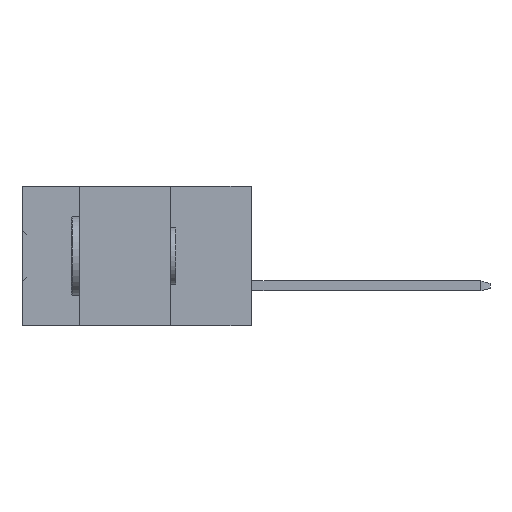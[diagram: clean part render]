
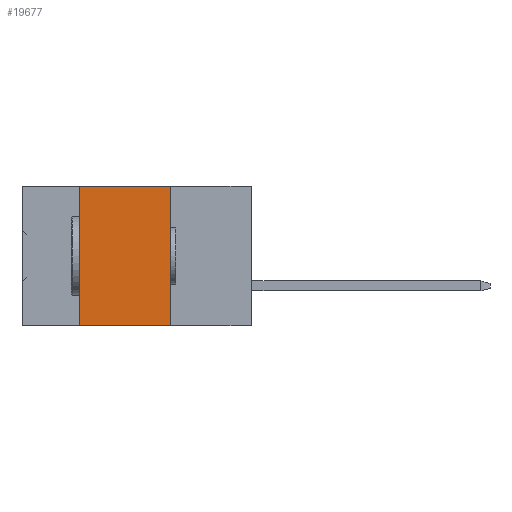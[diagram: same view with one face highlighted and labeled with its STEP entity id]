
A CAD part, left-side view. The second image highlights one B-rep face of the part: STEP entity #19677.
In plain terms, the highlighted planar face has unit normal (-1, 0, 0).
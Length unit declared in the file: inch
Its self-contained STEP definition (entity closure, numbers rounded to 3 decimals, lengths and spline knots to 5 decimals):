
#2339 = CARTESIAN_POINT ( 'NONE',  ( 0., 0.54, 0. ) ) ;
#2583 = AXIS2_PLACEMENT_3D ( 'NONE', #28787, #11927, #6808 ) ;
#3041 = CARTESIAN_POINT ( 'NONE',  ( 0., 0.54, -0.437 ) ) ;
#3697 = DIRECTION ( 'NONE',  ( 0., -1., 0. ) ) ;
#3862 = CARTESIAN_POINT ( 'NONE',  ( 0., 0.72, 0. ) ) ;
#4783 = LINE ( 'NONE', #19678, #19784 ) ;
#5439 = EDGE_CURVE ( 'NONE', #28182, #17520, #30820, .T. ) ;
#6808 = DIRECTION ( 'NONE',  ( 0., 0., -1. ) ) ;
#7467 = VERTEX_POINT ( 'NONE', #27757 ) ;
#9527 = EDGE_CURVE ( 'NONE', #17520, #7467, #4783, .T. ) ;
#10550 = EDGE_CURVE ( 'NONE', #27519, #7467, #31302, .T. ) ;
#11927 = DIRECTION ( 'NONE',  ( 1., 0., 0. ) ) ;
#12416 = ORIENTED_EDGE ( 'NONE', *, *, #9527, .F. ) ;
#12766 = CARTESIAN_POINT ( 'NONE',  ( 0., 0.54, -0.437 ) ) ;
#16402 = VECTOR ( 'NONE', #20463, 39.37008 ) ;
#17217 = ORIENTED_EDGE ( 'NONE', *, *, #10550, .T. ) ;
#17520 = VERTEX_POINT ( 'NONE', #27110 ) ;
#18548 = ORIENTED_EDGE ( 'NONE', *, *, #5439, .F. ) ;
#18601 = EDGE_LOOP ( 'NONE', ( #12416, #18548, #31200, #17217 ) ) ;
#18939 = EDGE_CURVE ( 'NONE', #27519, #28182, #20312, .T. ) ;
#18940 = DIRECTION ( 'NONE',  ( 0., -1., 0. ) ) ;
#19677 = ADVANCED_FACE ( 'NONE', ( #28937 ), #31674, .F. ) ;
#19678 = CARTESIAN_POINT ( 'NONE',  ( 0., 0.254, -0.437 ) ) ;
#19784 = VECTOR ( 'NONE', #24196, 39.37008 ) ;
#20312 = LINE ( 'NONE', #12766, #16402 ) ;
#20463 = DIRECTION ( 'NONE',  ( 0., 0., 1. ) ) ;
#21687 = VECTOR ( 'NONE', #3697, 39.37008 ) ;
#24196 = DIRECTION ( 'NONE',  ( 0., 0., -1. ) ) ;
#24388 = CARTESIAN_POINT ( 'NONE',  ( 0., 0.72, -0.437 ) ) ;
#24405 = VECTOR ( 'NONE', #18940, 39.37008 ) ;
#27110 = CARTESIAN_POINT ( 'NONE',  ( 0., 0.254, 0. ) ) ;
#27519 = VERTEX_POINT ( 'NONE', #3041 ) ;
#27757 = CARTESIAN_POINT ( 'NONE',  ( 0., 0.254, -0.437 ) ) ;
#28182 = VERTEX_POINT ( 'NONE', #2339 ) ;
#28787 = CARTESIAN_POINT ( 'NONE',  ( 0., 0.72, 0. ) ) ;
#28937 = FACE_OUTER_BOUND ( 'NONE', #18601, .T. ) ;
#30820 = LINE ( 'NONE', #3862, #21687 ) ;
#31200 = ORIENTED_EDGE ( 'NONE', *, *, #18939, .F. ) ;
#31302 = LINE ( 'NONE', #24388, #24405 ) ;
#31674 = PLANE ( 'NONE',  #2583 ) ;
